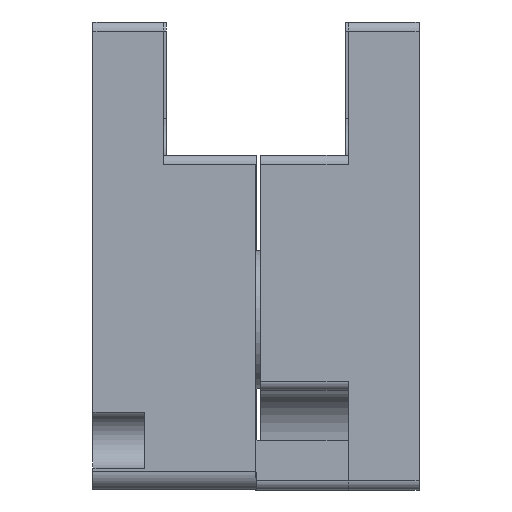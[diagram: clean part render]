
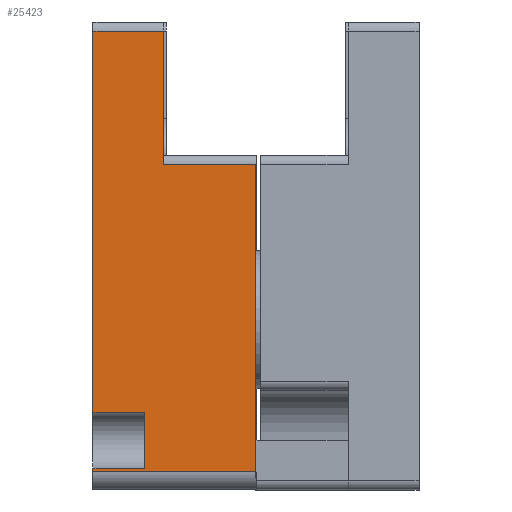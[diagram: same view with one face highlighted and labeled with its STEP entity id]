
A CAD part, left-side view. The second image highlights one B-rep face of the part: STEP entity #25423.
In plain terms, the highlighted planar face has unit normal (-1, 0, 0).
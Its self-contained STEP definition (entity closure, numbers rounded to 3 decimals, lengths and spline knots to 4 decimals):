
#2094=PLANE('',#26905);
#2807=FACE_OUTER_BOUND('',#4244,.T.);
#4244=EDGE_LOOP('',(#17573,#17574,#17575,#17576,#17577,#17578,#17579,#17580,
#17581,#17582));
#5857=LINE('',#32458,#8316);
#5858=LINE('',#32461,#8317);
#5859=LINE('',#32463,#8318);
#5860=LINE('',#32465,#8319);
#5861=LINE('',#32467,#8320);
#5862=LINE('',#32469,#8321);
#5863=LINE('',#32471,#8322);
#5864=LINE('',#32473,#8323);
#5865=LINE('',#32475,#8324);
#5866=LINE('',#32476,#8325);
#8316=VECTOR('',#27996,0.3937);
#8317=VECTOR('',#27999,0.3937);
#8318=VECTOR('',#28000,0.3937);
#8319=VECTOR('',#28001,0.3937);
#8320=VECTOR('',#28002,0.3937);
#8321=VECTOR('',#28003,0.3937);
#8322=VECTOR('',#28004,0.3937);
#8323=VECTOR('',#28005,0.3937);
#8324=VECTOR('',#28006,0.3937);
#8325=VECTOR('',#28007,0.3937);
#10984=VERTEX_POINT('',#32451);
#10987=VERTEX_POINT('',#32456);
#10988=VERTEX_POINT('',#32460);
#10989=VERTEX_POINT('',#32462);
#10990=VERTEX_POINT('',#32464);
#10991=VERTEX_POINT('',#32466);
#10992=VERTEX_POINT('',#32468);
#10993=VERTEX_POINT('',#32470);
#10994=VERTEX_POINT('',#32472);
#10995=VERTEX_POINT('',#32474);
#13621=EDGE_CURVE('',#10987,#10984,#5857,.T.);
#13622=EDGE_CURVE('',#10988,#10987,#5858,.T.);
#13623=EDGE_CURVE('',#10989,#10988,#5859,.T.);
#13624=EDGE_CURVE('',#10989,#10990,#5860,.T.);
#13625=EDGE_CURVE('',#10990,#10991,#5861,.T.);
#13626=EDGE_CURVE('',#10991,#10992,#5862,.T.);
#13627=EDGE_CURVE('',#10992,#10993,#5863,.T.);
#13628=EDGE_CURVE('',#10993,#10994,#5864,.T.);
#13629=EDGE_CURVE('',#10995,#10994,#5865,.T.);
#13630=EDGE_CURVE('',#10995,#10984,#5866,.T.);
#17573=ORIENTED_EDGE('',*,*,#13621,.F.);
#17574=ORIENTED_EDGE('',*,*,#13622,.F.);
#17575=ORIENTED_EDGE('',*,*,#13623,.F.);
#17576=ORIENTED_EDGE('',*,*,#13624,.T.);
#17577=ORIENTED_EDGE('',*,*,#13625,.T.);
#17578=ORIENTED_EDGE('',*,*,#13626,.T.);
#17579=ORIENTED_EDGE('',*,*,#13627,.T.);
#17580=ORIENTED_EDGE('',*,*,#13628,.T.);
#17581=ORIENTED_EDGE('',*,*,#13629,.F.);
#17582=ORIENTED_EDGE('',*,*,#13630,.T.);
#25423=ADVANCED_FACE('',(#2807),#2094,.T.);
#26905=AXIS2_PLACEMENT_3D('',#32459,#27997,#27998);
#27996=DIRECTION('',(0.,-1.,0.));
#27997=DIRECTION('center_axis',(-1.,0.,0.));
#27998=DIRECTION('ref_axis',(0.,0.,
-1.));
#27999=DIRECTION('',(0.,0.,-1.));
#28000=DIRECTION('',(0.,-1.,0.));
#28001=DIRECTION('',(0.,0.,-1.));
#28002=DIRECTION('',(0.,-1.,0.));
#28003=DIRECTION('',(0.,0.,-1.));
#28004=DIRECTION('',(0.,1.,0.));
#28005=DIRECTION('',(0.,0.,-1.));
#28006=DIRECTION('',(0.,1.,0.));
#28007=DIRECTION('',(0.,0.,1.));
#32451=CARTESIAN_POINT('',(-0.5965,0.,-0.8963));
#32456=CARTESIAN_POINT('',(-0.5965,0.3937,-0.8963));
#32458=CARTESIAN_POINT('',(-0.5965,0.5452,-0.8963));
#32459=CARTESIAN_POINT('Origin',(-0.5965,0.6968,-0.288));
#32460=CARTESIAN_POINT('',(-0.5965,0.3937,-0.3273));
#32461=CARTESIAN_POINT('',(-0.5965,0.3937,-0.288));
#32462=CARTESIAN_POINT('',(-0.5965,0.6968,-0.3273));
#32463=CARTESIAN_POINT('',(-0.5965,0.6968,-0.3273));
#32464=CARTESIAN_POINT('',(-0.5965,0.6968,-1.9548));
#32465=CARTESIAN_POINT('',(-0.5965,0.6968,-0.288));
#32466=CARTESIAN_POINT('',(-0.5965,0.4755,-1.9548));
#32467=CARTESIAN_POINT('',(-0.5965,0.6968,-1.9548));
#32468=CARTESIAN_POINT('',(-0.5965,0.4755,-2.1961));
#32469=CARTESIAN_POINT('',(-0.5965,0.4755,-1.1817));
#32470=CARTESIAN_POINT('',(-0.5965,0.6968,-2.1961));
#32471=CARTESIAN_POINT('',(-0.5965,0.6968,-2.1961));
#32472=CARTESIAN_POINT('',(-0.5965,0.6968,-2.209));
#32473=CARTESIAN_POINT('',(-0.5965,0.6968,-0.288));
#32474=CARTESIAN_POINT('',(-0.5965,0.,-2.209));
#32475=CARTESIAN_POINT('',(-0.5965,0.6968,-2.209));
#32476=CARTESIAN_POINT('',(-0.5965,0.,-1.196));
